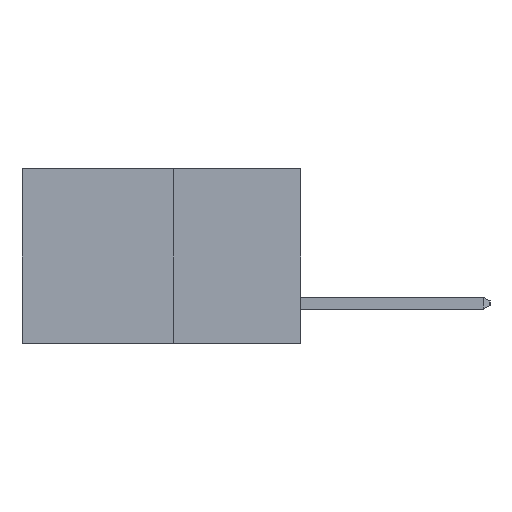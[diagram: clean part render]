
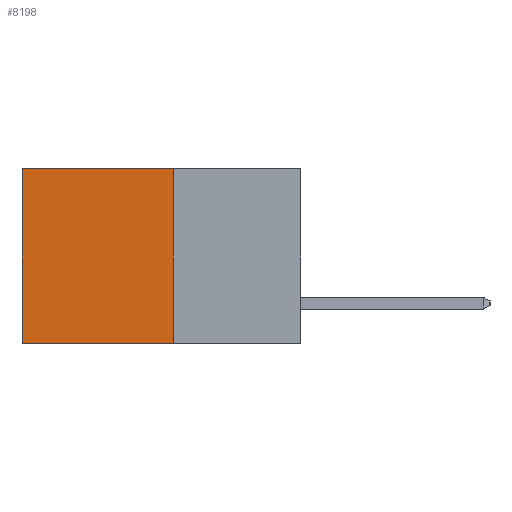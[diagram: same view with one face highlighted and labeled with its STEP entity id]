
A CAD part, left-side view. The second image highlights one B-rep face of the part: STEP entity #8198.
In plain terms, the highlighted planar face has unit normal (-1, 0, 0).
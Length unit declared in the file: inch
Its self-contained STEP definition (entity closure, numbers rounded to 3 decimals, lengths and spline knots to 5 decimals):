
#192 = DIRECTION ( 'NONE',  ( 0., 1., 0. ) ) ;
#684 = LINE ( 'NONE', #4053, #4125 ) ;
#1419 = CARTESIAN_POINT ( 'NONE',  ( 0.277, 0.59, 0. ) ) ;
#3172 = VERTEX_POINT ( 'NONE', #21653 ) ;
#4053 = CARTESIAN_POINT ( 'NONE',  ( 0.277, 0.27, -0.37 ) ) ;
#4125 = VECTOR ( 'NONE', #5818, 39.37008 ) ;
#4844 = CARTESIAN_POINT ( 'NONE',  ( 0.277, 0.59, -0.37 ) ) ;
#5818 = DIRECTION ( 'NONE',  ( 0., 1., 0. ) ) ;
#5956 = FACE_OUTER_BOUND ( 'NONE', #12964, .T. ) ;
#6597 = DIRECTION ( 'NONE',  ( 0., 0., -1. ) ) ;
#6749 = ORIENTED_EDGE ( 'NONE', *, *, #19738, .T. ) ;
#6918 = ORIENTED_EDGE ( 'NONE', *, *, #9829, .T. ) ;
#6934 = VECTOR ( 'NONE', #6597, 39.37008 ) ;
#8198 = ADVANCED_FACE ( 'NONE', ( #5956 ), #12270, .F. ) ;
#9771 = VECTOR ( 'NONE', #192, 39.37008 ) ;
#9829 = EDGE_CURVE ( 'NONE', #10473, #20021, #15820, .T. ) ;
#10271 = CARTESIAN_POINT ( 'NONE',  ( 0.277, 0.27, 0. ) ) ;
#10473 = VERTEX_POINT ( 'NONE', #1419 ) ;
#10764 = LINE ( 'NONE', #17750, #19204 ) ;
#10900 = CARTESIAN_POINT ( 'NONE',  ( 0.277, 0.59, -0.37 ) ) ;
#11283 = CARTESIAN_POINT ( 'NONE',  ( 0.277, 0.27, -0.37 ) ) ;
#12053 = EDGE_CURVE ( 'NONE', #17793, #20021, #684, .T. ) ;
#12270 = PLANE ( 'NONE',  #20861 ) ;
#12964 = EDGE_LOOP ( 'NONE', ( #6918, #18737, #14128, #6749 ) ) ;
#14084 = EDGE_CURVE ( 'NONE', #3172, #17793, #10764, .T. ) ;
#14128 = ORIENTED_EDGE ( 'NONE', *, *, #14084, .F. ) ;
#15393 = DIRECTION ( 'NONE',  ( 0., 0., -1. ) ) ;
#15473 = DIRECTION ( 'NONE',  ( 1., 0., 0. ) ) ;
#15820 = LINE ( 'NONE', #4844, #6934 ) ;
#17750 = CARTESIAN_POINT ( 'NONE',  ( 0.277, 0.27, -0.37 ) ) ;
#17793 = VERTEX_POINT ( 'NONE', #11283 ) ;
#18699 = LINE ( 'NONE', #10271, #9771 ) ;
#18737 = ORIENTED_EDGE ( 'NONE', *, *, #12053, .F. ) ;
#19204 = VECTOR ( 'NONE', #19417, 39.37008 ) ;
#19417 = DIRECTION ( 'NONE',  ( 0., 0., -1. ) ) ;
#19738 = EDGE_CURVE ( 'NONE', #3172, #10473, #18699, .T. ) ;
#20021 = VERTEX_POINT ( 'NONE', #10900 ) ;
#20345 = CARTESIAN_POINT ( 'NONE',  ( 0.277, 0.27, -0.37 ) ) ;
#20861 = AXIS2_PLACEMENT_3D ( 'NONE', #20345, #15473, #15393 ) ;
#21653 = CARTESIAN_POINT ( 'NONE',  ( 0.277, 0.27, 0. ) ) ;
